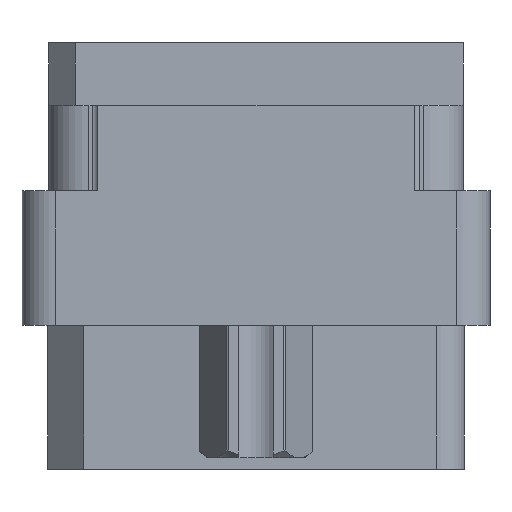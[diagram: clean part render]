
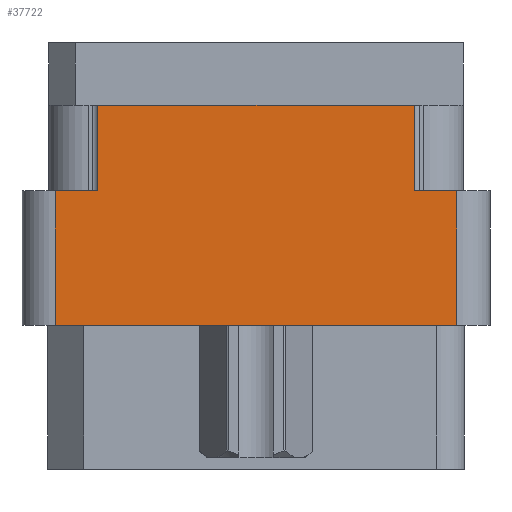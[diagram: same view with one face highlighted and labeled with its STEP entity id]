
A CAD part, left-side view. The second image highlights one B-rep face of the part: STEP entity #37722.
In plain terms, the highlighted planar face has unit normal (-1, 0, 0).
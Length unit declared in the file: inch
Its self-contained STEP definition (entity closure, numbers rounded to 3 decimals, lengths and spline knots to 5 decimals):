
#120 = ORIENTED_EDGE ( 'NONE', *, *, #37389, .F. ) ;
#577 = EDGE_CURVE ( 'NONE', #27628, #15928, #11294, .T. ) ;
#845 = EDGE_CURVE ( 'NONE', #24836, #3959, #3359, .T. ) ;
#1349 = DIRECTION ( 'NONE',  ( 0., 0., 1. ) ) ;
#1450 = CARTESIAN_POINT ( 'NONE',  ( -1., 0.296, -0.117 ) ) ;
#1566 = LINE ( 'NONE', #33051, #34797 ) ;
#1789 = ORIENTED_EDGE ( 'NONE', *, *, #11504, .F. ) ;
#3198 = DIRECTION ( 'NONE',  ( 0., 1., 0. ) ) ;
#3359 = LINE ( 'NONE', #35704, #12273 ) ;
#3693 = VERTEX_POINT ( 'NONE', #32778 ) ;
#3959 = VERTEX_POINT ( 'NONE', #19357 ) ;
#4322 = CARTESIAN_POINT ( 'NONE',  ( -1., 0.296, -0.277 ) ) ;
#4908 = CARTESIAN_POINT ( 'NONE',  ( -1., -0.376, -0.529 ) ) ;
#5276 = LINE ( 'NONE', #11132, #10639 ) ;
#7038 = DIRECTION ( 'NONE',  ( 0., 0., 1. ) ) ;
#7506 = EDGE_CURVE ( 'NONE', #26350, #26007, #26664, .T. ) ;
#10473 = DIRECTION ( 'NONE',  ( 0., -1., 0. ) ) ;
#10639 = VECTOR ( 'NONE', #36616, 39.37008 ) ;
#10689 = CARTESIAN_POINT ( 'NONE',  ( -1., -0.296, -0.277 ) ) ;
#11132 = CARTESIAN_POINT ( 'NONE',  ( -1., 0.438, -0.117 ) ) ;
#11294 = LINE ( 'NONE', #26534, #18900 ) ;
#11328 = AXIS2_PLACEMENT_3D ( 'NONE', #38157, #19333, #38766 ) ;
#11504 = EDGE_CURVE ( 'NONE', #24836, #15928, #32407, .T. ) ;
#12273 = VECTOR ( 'NONE', #22753, 39.37008 ) ;
#13133 = EDGE_CURVE ( 'NONE', #3693, #26350, #22691, .T. ) ;
#15102 = ORIENTED_EDGE ( 'NONE', *, *, #845, .T. ) ;
#15825 = VERTEX_POINT ( 'NONE', #1450 ) ;
#15928 = VERTEX_POINT ( 'NONE', #27669 ) ;
#16234 = CARTESIAN_POINT ( 'NONE',  ( -1., 0.438, -0.277 ) ) ;
#16849 = DIRECTION ( 'NONE',  ( 0., -1., 0. ) ) ;
#18199 = ORIENTED_EDGE ( 'NONE', *, *, #7506, .F. ) ;
#18900 = VECTOR ( 'NONE', #36578, 39.37008 ) ;
#19333 = DIRECTION ( 'NONE',  ( -1., 0., 0. ) ) ;
#19357 = CARTESIAN_POINT ( 'NONE',  ( -1., -0.296, -0.117 ) ) ;
#22173 = CARTESIAN_POINT ( 'NONE',  ( -1., -0.376, -0.529 ) ) ;
#22449 = ORIENTED_EDGE ( 'NONE', *, *, #13133, .F. ) ;
#22581 = VECTOR ( 'NONE', #3198, 39.37008 ) ;
#22691 = LINE ( 'NONE', #41069, #40787 ) ;
#22753 = DIRECTION ( 'NONE',  ( 0., 0., 1. ) ) ;
#23094 = PLANE ( 'NONE',  #11328 ) ;
#23681 = EDGE_CURVE ( 'NONE', #27628, #3693, #25301, .T. ) ;
#24836 = VERTEX_POINT ( 'NONE', #29478 ) ;
#25301 = LINE ( 'NONE', #22173, #22581 ) ;
#25570 = CARTESIAN_POINT ( 'NONE',  ( -1., 0.376, -0.277 ) ) ;
#26007 = VERTEX_POINT ( 'NONE', #4322 ) ;
#26350 = VERTEX_POINT ( 'NONE', #25570 ) ;
#26534 = CARTESIAN_POINT ( 'NONE',  ( -1., -0.376, -0.798 ) ) ;
#26664 = LINE ( 'NONE', #16234, #39691 ) ;
#27628 = VERTEX_POINT ( 'NONE', #4908 ) ;
#27669 = CARTESIAN_POINT ( 'NONE',  ( -1., -0.376, -0.277 ) ) ;
#28744 = FACE_OUTER_BOUND ( 'NONE', #37145, .T. ) ;
#29478 = CARTESIAN_POINT ( 'NONE',  ( -1., -0.296, -0.277 ) ) ;
#30286 = ORIENTED_EDGE ( 'NONE', *, *, #577, .T. ) ;
#32355 = VECTOR ( 'NONE', #10473, 39.37008 ) ;
#32391 = ORIENTED_EDGE ( 'NONE', *, *, #23681, .F. ) ;
#32407 = LINE ( 'NONE', #10689, #32355 ) ;
#32778 = CARTESIAN_POINT ( 'NONE',  ( -1., 0.376, -0.529 ) ) ;
#33051 = CARTESIAN_POINT ( 'NONE',  ( -1., 0.296, -0.277 ) ) ;
#34797 = VECTOR ( 'NONE', #1349, 39.37008 ) ;
#35704 = CARTESIAN_POINT ( 'NONE',  ( -1., -0.296, -0.277 ) ) ;
#36578 = DIRECTION ( 'NONE',  ( 0., 0., 1. ) ) ;
#36616 = DIRECTION ( 'NONE',  ( 0., -1., 0. ) ) ;
#37145 = EDGE_LOOP ( 'NONE', ( #22449, #32391, #30286, #1789, #15102, #120, #40572, #18199 ) ) ;
#37389 = EDGE_CURVE ( 'NONE', #15825, #3959, #5276, .T. ) ;
#37722 = ADVANCED_FACE ( 'NONE', ( #28744 ), #23094, .T. ) ;
#38157 = CARTESIAN_POINT ( 'NONE',  ( -1., -0.376, -0.798 ) ) ;
#38766 = DIRECTION ( 'NONE',  ( 0., 0., 1. ) ) ;
#39691 = VECTOR ( 'NONE', #16849, 39.37008 ) ;
#40333 = EDGE_CURVE ( 'NONE', #26007, #15825, #1566, .T. ) ;
#40572 = ORIENTED_EDGE ( 'NONE', *, *, #40333, .F. ) ;
#40787 = VECTOR ( 'NONE', #7038, 39.37008 ) ;
#41069 = CARTESIAN_POINT ( 'NONE',  ( -1., 0.376, -0.798 ) ) ;
